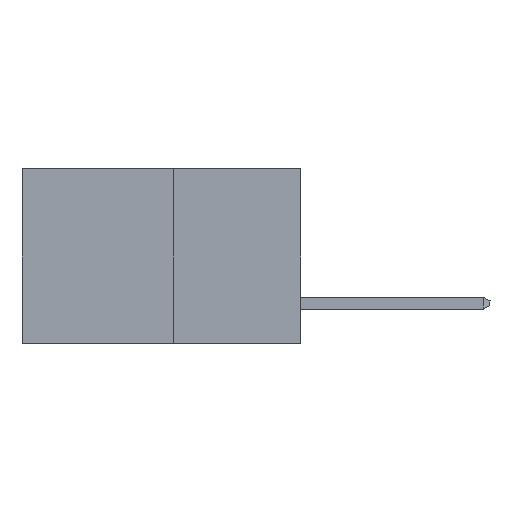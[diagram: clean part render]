
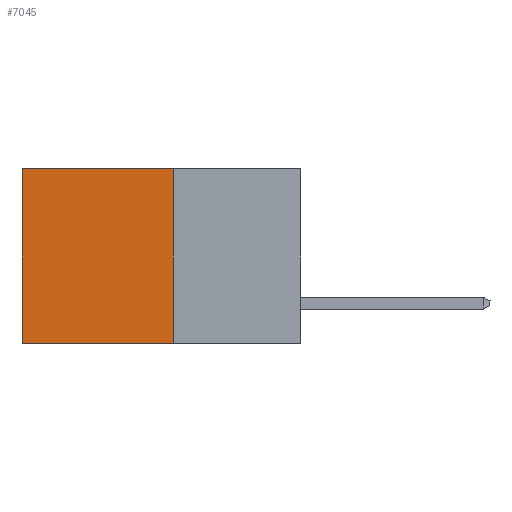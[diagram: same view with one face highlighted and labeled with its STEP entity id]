
A CAD part, left-side view. The second image highlights one B-rep face of the part: STEP entity #7045.
In plain terms, the highlighted planar face has unit normal (-1, 0, 0).
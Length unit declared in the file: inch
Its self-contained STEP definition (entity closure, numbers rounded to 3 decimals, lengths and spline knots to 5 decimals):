
#91 = CARTESIAN_POINT ( 'NONE',  ( 0.277, 0.27, -0.37 ) ) ;
#170 = EDGE_CURVE ( 'NONE', #10452, #1673, #9306, .T. ) ;
#402 = DIRECTION ( 'NONE',  ( 0., 0., -1. ) ) ;
#745 = DIRECTION ( 'NONE',  ( 0., 0., -1. ) ) ;
#762 = CARTESIAN_POINT ( 'NONE',  ( 0.277, 0.27, -0.37 ) ) ;
#1673 = VERTEX_POINT ( 'NONE', #1724 ) ;
#1724 = CARTESIAN_POINT ( 'NONE',  ( 0.277, 0.59, 0. ) ) ;
#2078 = ORIENTED_EDGE ( 'NONE', *, *, #8255, .F. ) ;
#2193 = FACE_OUTER_BOUND ( 'NONE', #4485, .T. ) ;
#2478 = CARTESIAN_POINT ( 'NONE',  ( 0.277, 0.59, -0.37 ) ) ;
#2934 = CARTESIAN_POINT ( 'NONE',  ( 0.277, 0.27, 0. ) ) ;
#3057 = CARTESIAN_POINT ( 'NONE',  ( 0.277, 0.27, 0. ) ) ;
#3343 = DIRECTION ( 'NONE',  ( 0., 1., 0. ) ) ;
#4226 = VECTOR ( 'NONE', #9872, 39.37008 ) ;
#4474 = VERTEX_POINT ( 'NONE', #8119 ) ;
#4485 = EDGE_LOOP ( 'NONE', ( #9088, #2078, #9957, #10402 ) ) ;
#5245 = EDGE_CURVE ( 'NONE', #10452, #6332, #6026, .T. ) ;
#6026 = LINE ( 'NONE', #762, #8810 ) ;
#6332 = VERTEX_POINT ( 'NONE', #12278 ) ;
#6543 = VECTOR ( 'NONE', #3343, 39.37008 ) ;
#6725 = LINE ( 'NONE', #91, #4226 ) ;
#7045 = ADVANCED_FACE ( 'NONE', ( #2193 ), #7923, .F. ) ;
#7093 = LINE ( 'NONE', #2478, #11753 ) ;
#7882 = DIRECTION ( 'NONE',  ( 0., 0., -1. ) ) ;
#7893 = DIRECTION ( 'NONE',  ( 1., 0., 0. ) ) ;
#7923 = PLANE ( 'NONE',  #12114 ) ;
#8111 = CARTESIAN_POINT ( 'NONE',  ( 0.277, 0.27, -0.37 ) ) ;
#8119 = CARTESIAN_POINT ( 'NONE',  ( 0.277, 0.59, -0.37 ) ) ;
#8255 = EDGE_CURVE ( 'NONE', #6332, #4474, #6725, .T. ) ;
#8810 = VECTOR ( 'NONE', #745, 39.37008 ) ;
#9088 = ORIENTED_EDGE ( 'NONE', *, *, #10015, .T. ) ;
#9306 = LINE ( 'NONE', #2934, #6543 ) ;
#9872 = DIRECTION ( 'NONE',  ( 0., 1., 0. ) ) ;
#9957 = ORIENTED_EDGE ( 'NONE', *, *, #5245, .F. ) ;
#10015 = EDGE_CURVE ( 'NONE', #1673, #4474, #7093, .T. ) ;
#10402 = ORIENTED_EDGE ( 'NONE', *, *, #170, .T. ) ;
#10452 = VERTEX_POINT ( 'NONE', #3057 ) ;
#11753 = VECTOR ( 'NONE', #402, 39.37008 ) ;
#12114 = AXIS2_PLACEMENT_3D ( 'NONE', #8111, #7893, #7882 ) ;
#12278 = CARTESIAN_POINT ( 'NONE',  ( 0.277, 0.27, -0.37 ) ) ;
